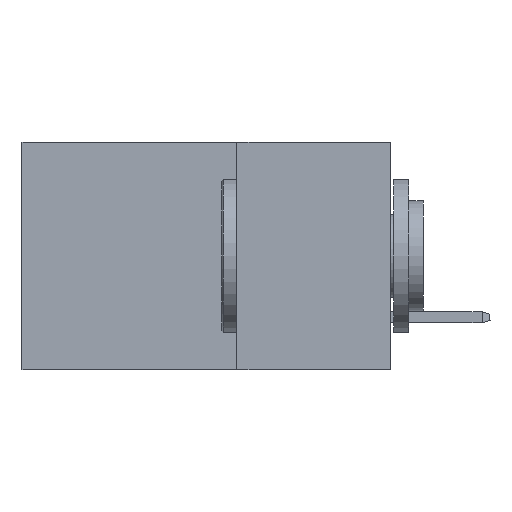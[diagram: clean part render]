
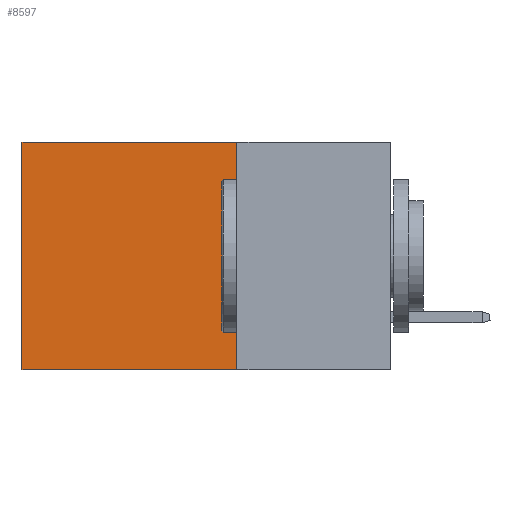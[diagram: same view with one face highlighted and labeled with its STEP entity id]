
A CAD part, left-side view. The second image highlights one B-rep face of the part: STEP entity #8597.
In plain terms, the highlighted planar face has unit normal (-1, 0, 0).
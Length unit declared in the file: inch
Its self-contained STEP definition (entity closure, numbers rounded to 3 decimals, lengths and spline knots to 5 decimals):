
#988 = VERTEX_POINT ( 'NONE', #2633 ) ;
#1696 = AXIS2_PLACEMENT_3D ( 'NONE', #35097, #38153, #27206 ) ;
#2633 = CARTESIAN_POINT ( 'NONE',  ( 0.2875, 0.25, -0.37 ) ) ;
#3967 = LINE ( 'NONE', #38106, #42075 ) ;
#5250 = DIRECTION ( 'NONE',  ( 0., 0., -1. ) ) ;
#5978 = LINE ( 'NONE', #30119, #19863 ) ;
#6320 = EDGE_CURVE ( 'NONE', #27020, #46596, #3967, .T. ) ;
#8597 = ADVANCED_FACE ( 'NONE', ( #45864 ), #23861, .F. ) ;
#8770 = CARTESIAN_POINT ( 'NONE',  ( 0.2875, 0.25, 0. ) ) ;
#10217 = LINE ( 'NONE', #38538, #28670 ) ;
#11360 = CARTESIAN_POINT ( 'NONE',  ( 0.2875, 0.6, -0.37 ) ) ;
#11950 = EDGE_LOOP ( 'NONE', ( #33213, #15357, #43677, #34253 ) ) ;
#13365 = DIRECTION ( 'NONE',  ( 0., 1., 0. ) ) ;
#15357 = ORIENTED_EDGE ( 'NONE', *, *, #25726, .F. ) ;
#16511 = DIRECTION ( 'NONE',  ( 0., 0., -1. ) ) ;
#18851 = VERTEX_POINT ( 'NONE', #11360 ) ;
#19863 = VECTOR ( 'NONE', #20630, 39.37008 ) ;
#20630 = DIRECTION ( 'NONE',  ( 0., 1., 0. ) ) ;
#20947 = EDGE_CURVE ( 'NONE', #46596, #18851, #10217, .T. ) ;
#21863 = EDGE_CURVE ( 'NONE', #27020, #988, #34606, .T. ) ;
#23861 = PLANE ( 'NONE',  #1696 ) ;
#25726 = EDGE_CURVE ( 'NONE', #988, #18851, #5978, .T. ) ;
#26391 = CARTESIAN_POINT ( 'NONE',  ( 0.2875, 0.6, 0. ) ) ;
#27020 = VERTEX_POINT ( 'NONE', #41241 ) ;
#27206 = DIRECTION ( 'NONE',  ( 0., 0., -1. ) ) ;
#28670 = VECTOR ( 'NONE', #16511, 39.37008 ) ;
#30119 = CARTESIAN_POINT ( 'NONE',  ( 0.2875, 0.25, -0.37 ) ) ;
#33213 = ORIENTED_EDGE ( 'NONE', *, *, #20947, .T. ) ;
#34253 = ORIENTED_EDGE ( 'NONE', *, *, #6320, .T. ) ;
#34606 = LINE ( 'NONE', #8770, #36347 ) ;
#35097 = CARTESIAN_POINT ( 'NONE',  ( 0.2875, 0.25, 0. ) ) ;
#36347 = VECTOR ( 'NONE', #5250, 39.37008 ) ;
#38106 = CARTESIAN_POINT ( 'NONE',  ( 0.2875, 0.25, 0. ) ) ;
#38153 = DIRECTION ( 'NONE',  ( 1., 0., 0. ) ) ;
#38538 = CARTESIAN_POINT ( 'NONE',  ( 0.2875, 0.6, 0. ) ) ;
#41241 = CARTESIAN_POINT ( 'NONE',  ( 0.2875, 0.25, 0. ) ) ;
#42075 = VECTOR ( 'NONE', #13365, 39.37008 ) ;
#43677 = ORIENTED_EDGE ( 'NONE', *, *, #21863, .F. ) ;
#45864 = FACE_OUTER_BOUND ( 'NONE', #11950, .T. ) ;
#46596 = VERTEX_POINT ( 'NONE', #26391 ) ;
